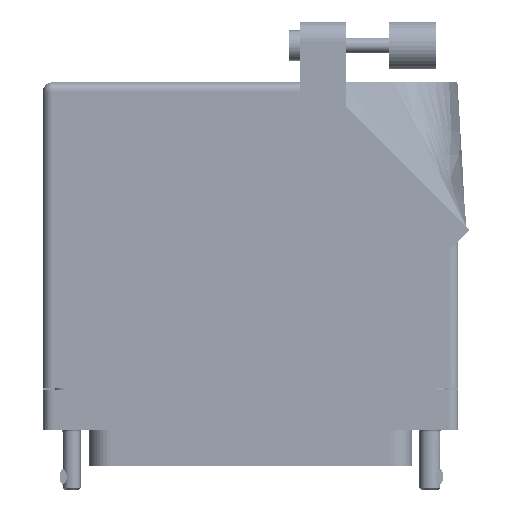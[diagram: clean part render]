
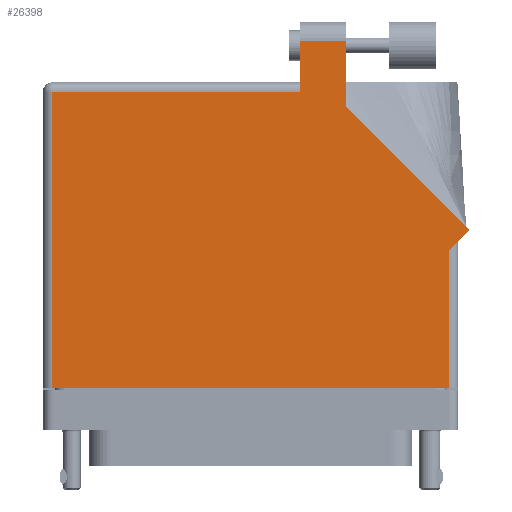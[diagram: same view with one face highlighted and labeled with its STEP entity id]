
A CAD part, front view. The second image highlights one B-rep face of the part: STEP entity #26398.
In plain terms, the highlighted face is planar.
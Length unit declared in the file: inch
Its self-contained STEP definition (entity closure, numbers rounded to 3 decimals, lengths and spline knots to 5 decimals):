
#1109 = CARTESIAN_POINT ( 'NONE',  ( 0.6345, 1.76442, 0.765 ) ) ;
#1139 = LINE ( 'NONE', #16551, #35917 ) ;
#2553 = ORIENTED_EDGE ( 'NONE', *, *, #59968, .T. ) ;
#2716 = CARTESIAN_POINT ( 'NONE',  ( 0.3275, 2.205, 0.765 ) ) ;
#2998 = VERTEX_POINT ( 'NONE', #1109 ) ;
#3642 = VERTEX_POINT ( 'NONE', #63846 ) ;
#5084 = CARTESIAN_POINT ( 'NONE',  ( -1.3155, -0.1, 0.765 ) ) ;
#7788 = VECTOR ( 'NONE', #95818, 39.37008 ) ;
#8816 = LINE ( 'NONE', #98009, #32392 ) ;
#9643 = ORIENTED_EDGE ( 'NONE', *, *, #29906, .T. ) ;
#9677 = DIRECTION ( 'NONE',  ( 0.707, 0.707, 0. ) ) ;
#11600 = ORIENTED_EDGE ( 'NONE', *, *, #12559, .T. ) ;
#12559 = EDGE_CURVE ( 'NONE', #2998, #35078, #1139, .T. ) ;
#16551 = CARTESIAN_POINT ( 'NONE',  ( 0.6345, 1.76442, 0.765 ) ) ;
#17363 = VECTOR ( 'NONE', #9677, 39.37008 ) ;
#19065 = EDGE_CURVE ( 'NONE', #3642, #79590, #53226, .T. ) ;
#19936 = EDGE_CURVE ( 'NONE', #35078, #47676, #95387, .T. ) ;
#21179 = EDGE_CURVE ( 'NONE', #69570, #2998, #66359, .T. ) ;
#21970 = VECTOR ( 'NONE', #48969, 39.37008 ) ;
#24401 = DIRECTION ( 'NONE',  ( 0., -1., 0. ) ) ;
#24588 = EDGE_CURVE ( 'NONE', #39851, #28415, #88077, .T. ) ;
#25312 = DIRECTION ( 'NONE',  ( 0., 1., 0. ) ) ;
#26398 = ADVANCED_FACE ( 'NONE', ( #58001 ), #74584, .F. ) ;
#28415 = VERTEX_POINT ( 'NONE', #49052 ) ;
#28419 = CARTESIAN_POINT ( 'NONE',  ( 0.6345, 2.205, 0.765 ) ) ;
#28901 = LINE ( 'NONE', #63797, #7788 ) ;
#29382 = VERTEX_POINT ( 'NONE', #92235 ) ;
#29906 = EDGE_CURVE ( 'NONE', #79590, #39851, #37827, .T. ) ;
#31058 = DIRECTION ( 'NONE',  ( -1., 0., 0. ) ) ;
#32203 = EDGE_CURVE ( 'NONE', #28415, #29382, #28901, .T. ) ;
#32392 = VECTOR ( 'NONE', #74026, 39.37008 ) ;
#34733 = EDGE_LOOP ( 'NONE', ( #11600, #68993, #2553, #71326, #9643, #77219, #85923, #79229, #67320 ) ) ;
#34966 = DIRECTION ( 'NONE',  ( 0., 0., -1. ) ) ;
#35078 = VERTEX_POINT ( 'NONE', #28419 ) ;
#35917 = VECTOR ( 'NONE', #25312, 39.37008 ) ;
#37827 = LINE ( 'NONE', #5084, #76467 ) ;
#38880 = CARTESIAN_POINT ( 'NONE',  ( 0.3275, 2.205, 0.765 ) ) ;
#38898 = DIRECTION ( 'NONE',  ( -0.707, 0.707, 0. ) ) ;
#39851 = VERTEX_POINT ( 'NONE', #41635 ) ;
#41635 = CARTESIAN_POINT ( 'NONE',  ( -1.3155, -0.1, 0.765 ) ) ;
#43945 = EDGE_CURVE ( 'NONE', #29382, #69570, #46155, .T. ) ;
#46155 = LINE ( 'NONE', #88235, #17363 ) ;
#46903 = CARTESIAN_POINT ( 'NONE',  ( 1.44821, 0.95071, 0.765 ) ) ;
#47064 = CARTESIAN_POINT ( 'NONE',  ( -1.3775, 1.868, 0.765 ) ) ;
#47646 = CARTESIAN_POINT ( 'NONE',  ( -1.3155, 1.868, 0.765 ) ) ;
#47676 = VERTEX_POINT ( 'NONE', #2716 ) ;
#48969 = DIRECTION ( 'NONE',  ( -1., 0., 0. ) ) ;
#49052 = CARTESIAN_POINT ( 'NONE',  ( 1.3155, -0.1, 0.765 ) ) ;
#50647 = DIRECTION ( 'NONE',  ( -1., 0., 0. ) ) ;
#50732 = VECTOR ( 'NONE', #31058, 39.37008 ) ;
#53226 = LINE ( 'NONE', #47064, #50732 ) ;
#58001 = FACE_OUTER_BOUND ( 'NONE', #34733, .T. ) ;
#58616 = CARTESIAN_POINT ( 'NONE',  ( -1.3775, 1.93, 0.765 ) ) ;
#59968 = EDGE_CURVE ( 'NONE', #47676, #3642, #8816, .T. ) ;
#63797 = CARTESIAN_POINT ( 'NONE',  ( 1.3155, 0.88, 0.765 ) ) ;
#63846 = CARTESIAN_POINT ( 'NONE',  ( 0.3275, 1.868, 0.765 ) ) ;
#66359 = LINE ( 'NONE', #46903, #101216 ) ;
#66969 = VECTOR ( 'NONE', #90128, 39.37008 ) ;
#67320 = ORIENTED_EDGE ( 'NONE', *, *, #21179, .T. ) ;
#68993 = ORIENTED_EDGE ( 'NONE', *, *, #19936, .T. ) ;
#69570 = VERTEX_POINT ( 'NONE', #95068 ) ;
#71326 = ORIENTED_EDGE ( 'NONE', *, *, #19065, .T. ) ;
#74026 = DIRECTION ( 'NONE',  ( 0., -1., 0. ) ) ;
#74584 = PLANE ( 'NONE',  #91985 ) ;
#76467 = VECTOR ( 'NONE', #24401, 39.37008 ) ;
#77219 = ORIENTED_EDGE ( 'NONE', *, *, #24588, .T. ) ;
#79229 = ORIENTED_EDGE ( 'NONE', *, *, #43945, .T. ) ;
#79590 = VERTEX_POINT ( 'NONE', #47646 ) ;
#85923 = ORIENTED_EDGE ( 'NONE', *, *, #32203, .T. ) ;
#88077 = LINE ( 'NONE', #96336, #66969 ) ;
#88235 = CARTESIAN_POINT ( 'NONE',  ( 1.3775, 0.88, 0.765 ) ) ;
#90128 = DIRECTION ( 'NONE',  ( 1., 0., 0. ) ) ;
#91985 = AXIS2_PLACEMENT_3D ( 'NONE', #58616, #34966, #50647 ) ;
#92235 = CARTESIAN_POINT ( 'NONE',  ( 1.3155, 0.818, 0.765 ) ) ;
#95068 = CARTESIAN_POINT ( 'NONE',  ( 1.44821, 0.95071, 0.765 ) ) ;
#95387 = LINE ( 'NONE', #38880, #21970 ) ;
#95818 = DIRECTION ( 'NONE',  ( 0., 1., 0. ) ) ;
#96336 = CARTESIAN_POINT ( 'NONE',  ( -1.3775, -0.1, 0.765 ) ) ;
#98009 = CARTESIAN_POINT ( 'NONE',  ( 0.3275, 1.93, 0.765 ) ) ;
#101216 = VECTOR ( 'NONE', #38898, 39.37008 ) ;
